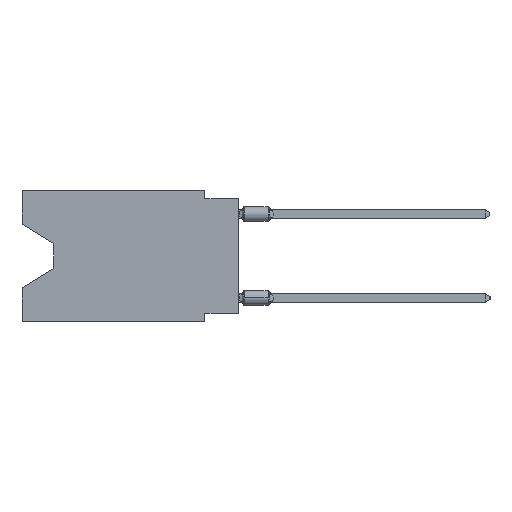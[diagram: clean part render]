
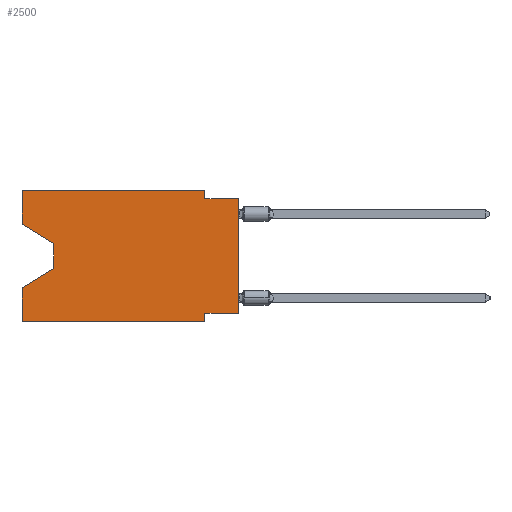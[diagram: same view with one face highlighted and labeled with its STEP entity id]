
A CAD part, left-side view. The second image highlights one B-rep face of the part: STEP entity #2500.
In plain terms, the highlighted planar face has unit normal (-1, 0, 0).
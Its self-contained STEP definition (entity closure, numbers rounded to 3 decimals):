
#330 = EDGE_CURVE ( 'NONE', #47916, #36860, #45121, .T. ) ;
#806 = DIRECTION ( 'NONE',  ( 0., -0.855, -0.519 ) ) ;
#878 = LINE ( 'NONE', #30142, #8201 ) ;
#2124 = CARTESIAN_POINT ( 'NONE',  ( 0., 0., -0.635 ) ) ;
#2500 = ADVANCED_FACE ( 'NONE', ( #40123 ), #15572, .F. ) ;
#3840 = EDGE_CURVE ( 'NONE', #32971, #43560, #42329, .T. ) ;
#3867 = VECTOR ( 'NONE', #806, 1000. ) ;
#4148 = CARTESIAN_POINT ( 'NONE',  ( 0., 16.383, 0. ) ) ;
#4662 = CARTESIAN_POINT ( 'NONE',  ( 0., 2.54, -9.906 ) ) ;
#6013 = CARTESIAN_POINT ( 'NONE',  ( 0., 16.383, 0. ) ) ;
#6305 = EDGE_CURVE ( 'NONE', #9527, #46567, #27440, .T. ) ;
#6564 = ORIENTED_EDGE ( 'NONE', *, *, #15710, .F. ) ;
#7385 = LINE ( 'NONE', #50823, #23589 ) ;
#8078 = ORIENTED_EDGE ( 'NONE', *, *, #13294, .F. ) ;
#8201 = VECTOR ( 'NONE', #8943, 1000. ) ;
#8817 = EDGE_CURVE ( 'NONE', #32971, #35040, #7385, .T. ) ;
#8943 = DIRECTION ( 'NONE',  ( 0., 0., -1. ) ) ;
#9527 = VERTEX_POINT ( 'NONE', #28162 ) ;
#9888 = VERTEX_POINT ( 'NONE', #2124 ) ;
#11196 = DIRECTION ( 'NONE',  ( 0., 0.855, -0.519 ) ) ;
#11776 = LINE ( 'NONE', #24609, #35412 ) ;
#11897 = CARTESIAN_POINT ( 'NONE',  ( 0., 0., -9.271 ) ) ;
#12016 = CARTESIAN_POINT ( 'NONE',  ( 0., 13.97, -5.893 ) ) ;
#13269 = ORIENTED_EDGE ( 'NONE', *, *, #38393, .F. ) ;
#13294 = EDGE_CURVE ( 'NONE', #31641, #26464, #26147, .T. ) ;
#13466 = VECTOR ( 'NONE', #23013, 1000. ) ;
#14277 = EDGE_LOOP ( 'NONE', ( #44206, #40451, #24097, #52653, #43073, #6564, #51419, #52630, #13269, #38870, #39947, #8078 ) ) ;
#14746 = DIRECTION ( 'NONE',  ( 0., 0., -1. ) ) ;
#15426 = LINE ( 'NONE', #32444, #19510 ) ;
#15572 = PLANE ( 'NONE',  #16006 ) ;
#15710 = EDGE_CURVE ( 'NONE', #36860, #35040, #11776, .T. ) ;
#16006 = AXIS2_PLACEMENT_3D ( 'NONE', #40401, #32309, #14746 ) ;
#16310 = CARTESIAN_POINT ( 'NONE',  ( 0., 2.54, -9.271 ) ) ;
#17974 = VECTOR ( 'NONE', #27717, 1000. ) ;
#18490 = CARTESIAN_POINT ( 'NONE',  ( 0., 16.383, 0. ) ) ;
#19510 = VECTOR ( 'NONE', #41080, 1000. ) ;
#20536 = VERTEX_POINT ( 'NONE', #37784 ) ;
#21064 = EDGE_CURVE ( 'NONE', #20536, #40114, #878, .T. ) ;
#23013 = DIRECTION ( 'NONE',  ( 0., -1., 0. ) ) ;
#23589 = VECTOR ( 'NONE', #32763, 1000. ) ;
#24097 = ORIENTED_EDGE ( 'NONE', *, *, #50985, .T. ) ;
#24418 = EDGE_CURVE ( 'NONE', #31641, #20536, #34800, .T. ) ;
#24609 = CARTESIAN_POINT ( 'NONE',  ( 0., 2.54, -9.906 ) ) ;
#25610 = DIRECTION ( 'NONE',  ( 0., 0., 1. ) ) ;
#26147 = LINE ( 'NONE', #47583, #49418 ) ;
#26464 = VERTEX_POINT ( 'NONE', #18490 ) ;
#27204 = LINE ( 'NONE', #6013, #13466 ) ;
#27440 = LINE ( 'NONE', #45525, #17974 ) ;
#27518 = CARTESIAN_POINT ( 'NONE',  ( 0., 2.54, -0.635 ) ) ;
#27717 = DIRECTION ( 'NONE',  ( 0., 0., -1. ) ) ;
#28090 = VECTOR ( 'NONE', #38637, 1000. ) ;
#28162 = CARTESIAN_POINT ( 'NONE',  ( 0., 2.54, 0. ) ) ;
#30142 = CARTESIAN_POINT ( 'NONE',  ( 0., 13.97, -4.013 ) ) ;
#31281 = CARTESIAN_POINT ( 'NONE',  ( 0., 0., 0. ) ) ;
#31641 = VERTEX_POINT ( 'NONE', #50078 ) ;
#32170 = VECTOR ( 'NONE', #34241, 1000. ) ;
#32309 = DIRECTION ( 'NONE',  ( 1., 0., 0. ) ) ;
#32444 = CARTESIAN_POINT ( 'NONE',  ( 0., 0., -0.635 ) ) ;
#32763 = DIRECTION ( 'NONE',  ( 0., -1., 0. ) ) ;
#32971 = VERTEX_POINT ( 'NONE', #41876 ) ;
#34241 = DIRECTION ( 'NONE',  ( 0., 0., 1. ) ) ;
#34249 = CARTESIAN_POINT ( 'NONE',  ( 0., 0., -9.271 ) ) ;
#34800 = LINE ( 'NONE', #39264, #3867 ) ;
#35040 = VERTEX_POINT ( 'NONE', #4662 ) ;
#35412 = VECTOR ( 'NONE', #41617, 1000. ) ;
#35469 = CARTESIAN_POINT ( 'NONE',  ( 0., 13.97, -5.893 ) ) ;
#36617 = EDGE_CURVE ( 'NONE', #26464, #9527, #27204, .T. ) ;
#36860 = VERTEX_POINT ( 'NONE', #16310 ) ;
#37784 = CARTESIAN_POINT ( 'NONE',  ( 0., 13.97, -4.013 ) ) ;
#38165 = VECTOR ( 'NONE', #11196, 1000. ) ;
#38166 = DIRECTION ( 'NONE',  ( 0., 1., 0. ) ) ;
#38393 = EDGE_CURVE ( 'NONE', #46567, #9888, #15426, .T. ) ;
#38637 = DIRECTION ( 'NONE',  ( 0., 0., 1. ) ) ;
#38870 = ORIENTED_EDGE ( 'NONE', *, *, #6305, .F. ) ;
#39264 = CARTESIAN_POINT ( 'NONE',  ( 0., 16.383, -2.546 ) ) ;
#39947 = ORIENTED_EDGE ( 'NONE', *, *, #36617, .F. ) ;
#40114 = VERTEX_POINT ( 'NONE', #12016 ) ;
#40123 = FACE_OUTER_BOUND ( 'NONE', #14277, .T. ) ;
#40401 = CARTESIAN_POINT ( 'NONE',  ( 0., 16.383, 0. ) ) ;
#40451 = ORIENTED_EDGE ( 'NONE', *, *, #21064, .T. ) ;
#41080 = DIRECTION ( 'NONE',  ( 0., -1., 0. ) ) ;
#41617 = DIRECTION ( 'NONE',  ( 0., 0., -1. ) ) ;
#41876 = CARTESIAN_POINT ( 'NONE',  ( 0., 16.383, -9.906 ) ) ;
#42329 = LINE ( 'NONE', #4148, #32170 ) ;
#42800 = LINE ( 'NONE', #31281, #28090 ) ;
#43073 = ORIENTED_EDGE ( 'NONE', *, *, #8817, .T. ) ;
#43560 = VERTEX_POINT ( 'NONE', #51535 ) ;
#44206 = ORIENTED_EDGE ( 'NONE', *, *, #24418, .T. ) ;
#44240 = VECTOR ( 'NONE', #38166, 1000. ) ;
#45121 = LINE ( 'NONE', #34249, #44240 ) ;
#45525 = CARTESIAN_POINT ( 'NONE',  ( 0., 2.54, 0. ) ) ;
#45658 = EDGE_CURVE ( 'NONE', #47916, #9888, #42800, .T. ) ;
#46567 = VERTEX_POINT ( 'NONE', #27518 ) ;
#47583 = CARTESIAN_POINT ( 'NONE',  ( 0., 16.383, 0. ) ) ;
#47916 = VERTEX_POINT ( 'NONE', #11897 ) ;
#49418 = VECTOR ( 'NONE', #25610, 1000. ) ;
#50078 = CARTESIAN_POINT ( 'NONE',  ( 0., 16.383, -2.546 ) ) ;
#50823 = CARTESIAN_POINT ( 'NONE',  ( 0., 16.383, -9.906 ) ) ;
#50985 = EDGE_CURVE ( 'NONE', #40114, #43560, #52408, .T. ) ;
#51419 = ORIENTED_EDGE ( 'NONE', *, *, #330, .F. ) ;
#51535 = CARTESIAN_POINT ( 'NONE',  ( 0., 16.383, -7.36 ) ) ;
#52408 = LINE ( 'NONE', #35469, #38165 ) ;
#52630 = ORIENTED_EDGE ( 'NONE', *, *, #45658, .T. ) ;
#52653 = ORIENTED_EDGE ( 'NONE', *, *, #3840, .F. ) ;
